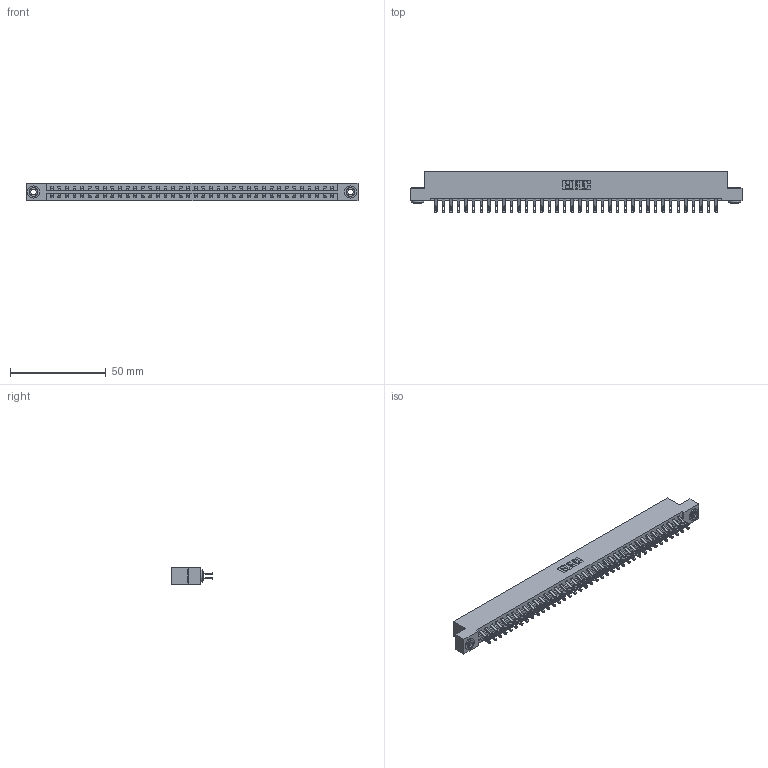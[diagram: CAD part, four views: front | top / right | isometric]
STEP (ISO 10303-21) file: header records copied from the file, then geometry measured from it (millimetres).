
FILE_DESCRIPTION (( 'STEP AP203' ), '1' );
FILE_NAME ('387-076-555-203.STEP', '2019-10-22T04:12:58', ( '' ), ( '' ), 'SwSTEP 2.0', 'SolidWorks 2016', '' );
FILE_SCHEMA (( 'CONFIG_CONTROL_DESIGN' ));
Length unit declared in the file: inch
Products named in the file (4): 387-076-555-203; 345-292-001_555 Tail; 337 Part_Flush Mounting Lugs - 0.156 Dia-TH; 345-250-002_345-250-002-102
Assembly tree (79 placements, depth 2):
  387-076-555-203
    337 Part_Flush Mounting Lugs - 0.156 Dia-TH
    345-292-001_555 Tail  x76
    345-250-002_345-250-002-102  x2
Bounding box: 173.58 x 21.47 x 9.4 mm (x, y, z)
Volume: 18480.2 mm3; surface area: 21908.2 mm2
Topology: 79 solids, 79 shells, 4712 faces, 14751 edges, 9830 vertices
Faces by surface type: plane 2816, cylinder 1888, cone 8
Entity records: 30956 total; most frequent: CARTESIAN_POINT 5227, ORIENTED_EDGE 5126, DIRECTION 4457, EDGE_CURVE 2563, VECTOR 2391, LINE 2391, VERTEX_POINT 1706, AXIS2_PLACEMENT_3D 1033
